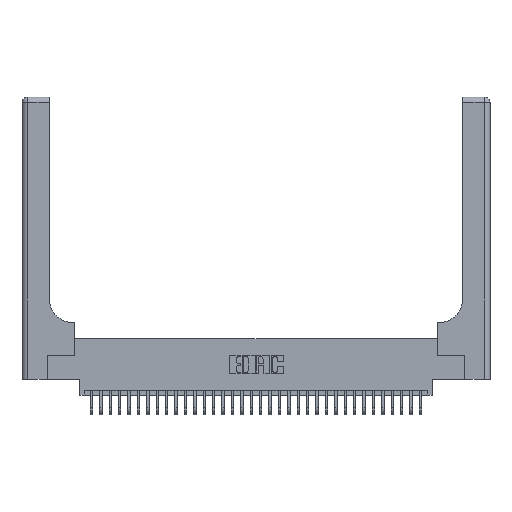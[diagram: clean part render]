
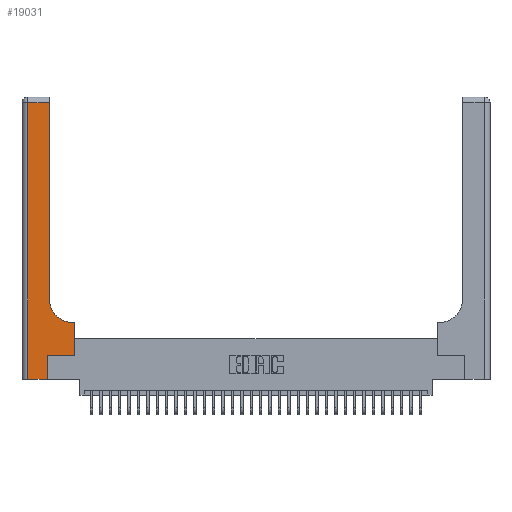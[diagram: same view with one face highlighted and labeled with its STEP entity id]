
A CAD part, top view. The second image highlights one B-rep face of the part: STEP entity #19031.
In plain terms, the highlighted planar face has unit normal (0, 0, 1).
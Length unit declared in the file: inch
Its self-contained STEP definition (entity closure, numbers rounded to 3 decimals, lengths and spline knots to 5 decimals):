
#273 = FACE_OUTER_BOUND ( 'NONE', #21590, .T. ) ;
#443 = VECTOR ( 'NONE', #35298, 39.37008 ) ;
#616 = VERTEX_POINT ( 'NONE', #33828 ) ;
#942 = LINE ( 'NONE', #1304, #19345 ) ;
#1304 = CARTESIAN_POINT ( 'NONE',  ( 0.5585, 0.25, 0.37 ) ) ;
#3097 = DIRECTION ( 'NONE',  ( -1., 0., 0. ) ) ;
#4459 = ORIENTED_EDGE ( 'NONE', *, *, #5936, .T. ) ;
#5669 = AXIS2_PLACEMENT_3D ( 'NONE', #12221, #7315, #23275 ) ;
#5936 = EDGE_CURVE ( 'NONE', #616, #35066, #35428, .T. ) ;
#6270 = CARTESIAN_POINT ( 'NONE',  ( 0.269, 0.25, 0.37 ) ) ;
#6644 = DIRECTION ( 'NONE',  ( 0., 1., 0. ) ) ;
#7315 = DIRECTION ( 'NONE',  ( 0., 0., -1. ) ) ;
#7500 = CARTESIAN_POINT ( 'NONE',  ( 0.2915, 2.94, 0.37 ) ) ;
#8588 = VECTOR ( 'NONE', #6644, 39.37008 ) ;
#8605 = CARTESIAN_POINT ( 'NONE',  ( 0., 3., 0.37 ) ) ;
#8863 = EDGE_CURVE ( 'NONE', #35066, #16015, #28000, .T. ) ;
#9413 = EDGE_CURVE ( 'NONE', #15476, #22063, #942, .T. ) ;
#9868 = EDGE_CURVE ( 'NONE', #22063, #11526, #15378, .T. ) ;
#10180 = LINE ( 'NONE', #29799, #34897 ) ;
#11483 = DIRECTION ( 'NONE',  ( 0., 0., -1. ) ) ;
#11526 = VERTEX_POINT ( 'NONE', #26499 ) ;
#12046 = AXIS2_PLACEMENT_3D ( 'NONE', #8605, #11483, #16973 ) ;
#12221 = CARTESIAN_POINT ( 'NONE',  ( 0.5415, 0.85, 0.37 ) ) ;
#12582 = DIRECTION ( 'NONE',  ( 1., 0., 0. ) ) ;
#14065 = CARTESIAN_POINT ( 'NONE',  ( 0.2915, 0.6, 0.37 ) ) ;
#14817 = DIRECTION ( 'NONE',  ( 1., 0., 0. ) ) ;
#15088 = CARTESIAN_POINT ( 'NONE',  ( 0.06, 3., 0.37 ) ) ;
#15378 = LINE ( 'NONE', #14065, #443 ) ;
#15400 = VERTEX_POINT ( 'NONE', #21319 ) ;
#15476 = VERTEX_POINT ( 'NONE', #35260 ) ;
#16015 = VERTEX_POINT ( 'NONE', #32055 ) ;
#16389 = VECTOR ( 'NONE', #20873, 39.37008 ) ;
#16973 = DIRECTION ( 'NONE',  ( -1., 0., 0. ) ) ;
#17461 = ORIENTED_EDGE ( 'NONE', *, *, #9868, .T. ) ;
#17611 = VECTOR ( 'NONE', #12582, 39.37008 ) ;
#19011 = EDGE_CURVE ( 'NONE', #21865, #616, #29079, .T. ) ;
#19031 = ADVANCED_FACE ( 'NONE', ( #273 ), #25324, .F. ) ;
#19345 = VECTOR ( 'NONE', #26131, 39.37008 ) ;
#20169 = ORIENTED_EDGE ( 'NONE', *, *, #25281, .T. ) ;
#20584 = EDGE_CURVE ( 'NONE', #23890, #15476, #10180, .T. ) ;
#20873 = DIRECTION ( 'NONE',  ( 0., 1., 0. ) ) ;
#21319 = CARTESIAN_POINT ( 'NONE',  ( 0.2915, 0.85, 0.37 ) ) ;
#21590 = EDGE_LOOP ( 'NONE', ( #35595, #22847, #4459, #31841, #20169, #27583, #22260, #17461, #34215 ) ) ;
#21724 = VECTOR ( 'NONE', #3097, 39.37008 ) ;
#21865 = VERTEX_POINT ( 'NONE', #7500 ) ;
#22063 = VERTEX_POINT ( 'NONE', #27507 ) ;
#22260 = ORIENTED_EDGE ( 'NONE', *, *, #9413, .T. ) ;
#22847 = ORIENTED_EDGE ( 'NONE', *, *, #19011, .T. ) ;
#23008 = CARTESIAN_POINT ( 'NONE',  ( 0.2915, 3., 0.37 ) ) ;
#23275 = DIRECTION ( 'NONE',  ( 1., 0., 0. ) ) ;
#23401 = EDGE_CURVE ( 'NONE', #11526, #15400, #29014, .T. ) ;
#23890 = VERTEX_POINT ( 'NONE', #6270 ) ;
#23900 = EDGE_CURVE ( 'NONE', #15400, #21865, #27273, .T. ) ;
#24991 = VECTOR ( 'NONE', #31968, 39.37008 ) ;
#25122 = CARTESIAN_POINT ( 'NONE',  ( 0.06, 0., 0.37 ) ) ;
#25281 = EDGE_CURVE ( 'NONE', #16015, #23890, #30305, .T. ) ;
#25324 = PLANE ( 'NONE',  #12046 ) ;
#26131 = DIRECTION ( 'NONE',  ( 0., 1., 0. ) ) ;
#26306 = CARTESIAN_POINT ( 'NONE',  ( 0., 0., 0.37 ) ) ;
#26499 = CARTESIAN_POINT ( 'NONE',  ( 0.5415, 0.6, 0.37 ) ) ;
#27273 = LINE ( 'NONE', #23008, #8588 ) ;
#27507 = CARTESIAN_POINT ( 'NONE',  ( 0.5585, 0.6, 0.37 ) ) ;
#27583 = ORIENTED_EDGE ( 'NONE', *, *, #20584, .T. ) ;
#28000 = LINE ( 'NONE', #26306, #17611 ) ;
#29014 = CIRCLE ( 'NONE', #5669, 0.25 ) ;
#29079 = LINE ( 'NONE', #31052, #21724 ) ;
#29799 = CARTESIAN_POINT ( 'NONE',  ( 0.269, 0.25, 0.37 ) ) ;
#30305 = LINE ( 'NONE', #34720, #16389 ) ;
#31052 = CARTESIAN_POINT ( 'NONE',  ( 0., 2.94, 0.37 ) ) ;
#31841 = ORIENTED_EDGE ( 'NONE', *, *, #8863, .T. ) ;
#31968 = DIRECTION ( 'NONE',  ( 0., -1., 0. ) ) ;
#32055 = CARTESIAN_POINT ( 'NONE',  ( 0.269, 0., 0.37 ) ) ;
#33828 = CARTESIAN_POINT ( 'NONE',  ( 0.06, 2.94, 0.37 ) ) ;
#34215 = ORIENTED_EDGE ( 'NONE', *, *, #23401, .T. ) ;
#34720 = CARTESIAN_POINT ( 'NONE',  ( 0.269, 0., 0.37 ) ) ;
#34897 = VECTOR ( 'NONE', #14817, 39.37008 ) ;
#35066 = VERTEX_POINT ( 'NONE', #25122 ) ;
#35260 = CARTESIAN_POINT ( 'NONE',  ( 0.5585, 0.25, 0.37 ) ) ;
#35298 = DIRECTION ( 'NONE',  ( -1., 0., 0. ) ) ;
#35428 = LINE ( 'NONE', #15088, #24991 ) ;
#35595 = ORIENTED_EDGE ( 'NONE', *, *, #23900, .T. ) ;
